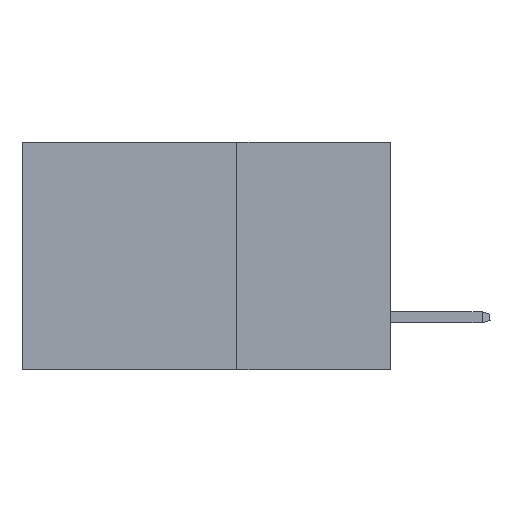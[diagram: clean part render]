
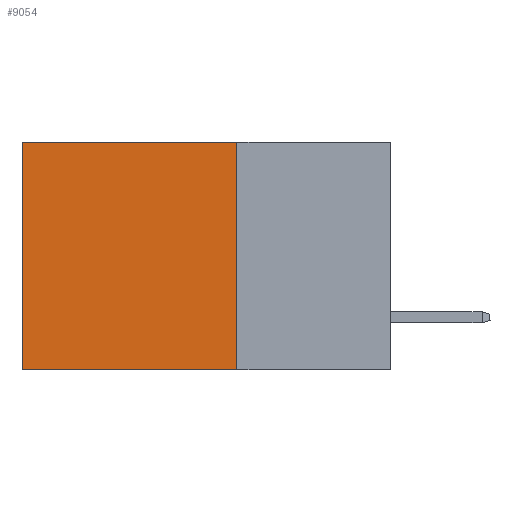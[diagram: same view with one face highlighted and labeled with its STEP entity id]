
A CAD part, left-side view. The second image highlights one B-rep face of the part: STEP entity #9054.
In plain terms, the highlighted planar face has unit normal (-1, 0, 0).
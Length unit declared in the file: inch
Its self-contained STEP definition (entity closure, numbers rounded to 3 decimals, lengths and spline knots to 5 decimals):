
#1440 = CARTESIAN_POINT ( 'NONE',  ( 0.2875, 0.25, -0.37 ) ) ;
#1980 = EDGE_CURVE ( 'NONE', #16479, #8188, #28522, .T. ) ;
#4041 = EDGE_CURVE ( 'NONE', #12181, #16479, #31221, .T. ) ;
#4742 = CARTESIAN_POINT ( 'NONE',  ( 0.2875, 0.6, 0. ) ) ;
#6953 = VECTOR ( 'NONE', #28530, 39.37008 ) ;
#8188 = VERTEX_POINT ( 'NONE', #31442 ) ;
#8459 = DIRECTION ( 'NONE',  ( 0., 1., 0. ) ) ;
#9054 = ADVANCED_FACE ( 'NONE', ( #12950 ), #14868, .F. ) ;
#11789 = DIRECTION ( 'NONE',  ( 1., 0., 0. ) ) ;
#12181 = VERTEX_POINT ( 'NONE', #28386 ) ;
#12402 = EDGE_CURVE ( 'NONE', #27942, #8188, #36370, .T. ) ;
#12950 = FACE_OUTER_BOUND ( 'NONE', #18592, .T. ) ;
#13764 = CARTESIAN_POINT ( 'NONE',  ( 0.2875, 0.25, -0.37 ) ) ;
#14868 = PLANE ( 'NONE',  #26939 ) ;
#15126 = DIRECTION ( 'NONE',  ( 0., 0., -1. ) ) ;
#15644 = LINE ( 'NONE', #32818, #37757 ) ;
#16479 = VERTEX_POINT ( 'NONE', #35509 ) ;
#18592 = EDGE_LOOP ( 'NONE', ( #41306, #42959, #38497, #30721 ) ) ;
#22044 = VECTOR ( 'NONE', #8459, 39.37008 ) ;
#23119 = CARTESIAN_POINT ( 'NONE',  ( 0.2875, 0.25, 0. ) ) ;
#26939 = AXIS2_PLACEMENT_3D ( 'NONE', #23119, #11789, #15126 ) ;
#27942 = VERTEX_POINT ( 'NONE', #13764 ) ;
#28386 = CARTESIAN_POINT ( 'NONE',  ( 0.2875, 0.25, 0. ) ) ;
#28522 = LINE ( 'NONE', #4742, #6953 ) ;
#28530 = DIRECTION ( 'NONE',  ( 0., 0., -1. ) ) ;
#30721 = ORIENTED_EDGE ( 'NONE', *, *, #4041, .T. ) ;
#30957 = VECTOR ( 'NONE', #43050, 39.37008 ) ;
#31221 = LINE ( 'NONE', #32557, #22044 ) ;
#31442 = CARTESIAN_POINT ( 'NONE',  ( 0.2875, 0.6, -0.37 ) ) ;
#32557 = CARTESIAN_POINT ( 'NONE',  ( 0.2875, 0.25, 0. ) ) ;
#32818 = CARTESIAN_POINT ( 'NONE',  ( 0.2875, 0.25, 0. ) ) ;
#34871 = EDGE_CURVE ( 'NONE', #12181, #27942, #15644, .T. ) ;
#35509 = CARTESIAN_POINT ( 'NONE',  ( 0.2875, 0.6, 0. ) ) ;
#36370 = LINE ( 'NONE', #1440, #30957 ) ;
#37757 = VECTOR ( 'NONE', #43265, 39.37008 ) ;
#38497 = ORIENTED_EDGE ( 'NONE', *, *, #34871, .F. ) ;
#41306 = ORIENTED_EDGE ( 'NONE', *, *, #1980, .T. ) ;
#42959 = ORIENTED_EDGE ( 'NONE', *, *, #12402, .F. ) ;
#43050 = DIRECTION ( 'NONE',  ( 0., 1., 0. ) ) ;
#43265 = DIRECTION ( 'NONE',  ( 0., 0., -1. ) ) ;
